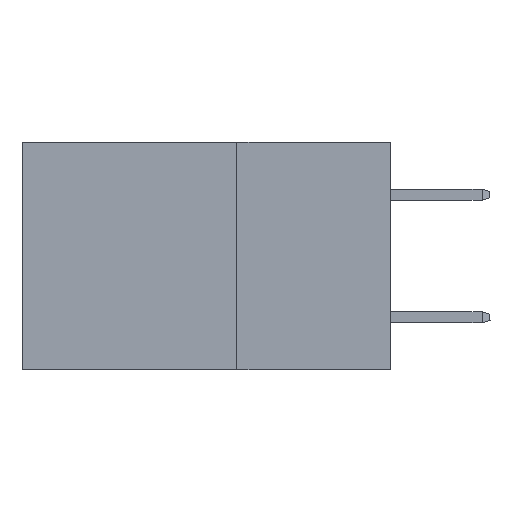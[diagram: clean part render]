
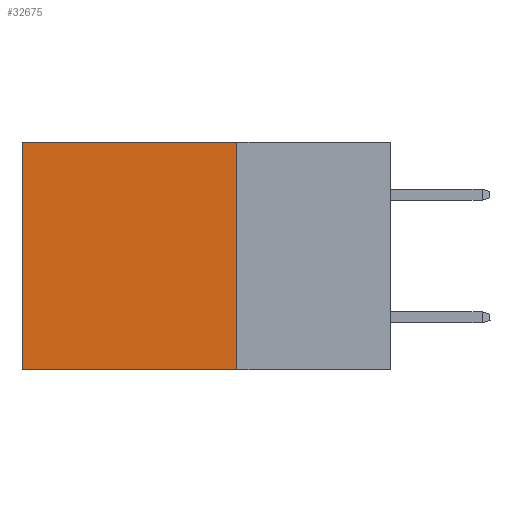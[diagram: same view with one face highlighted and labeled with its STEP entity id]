
A CAD part, left-side view. The second image highlights one B-rep face of the part: STEP entity #32675.
In plain terms, the highlighted planar face has unit normal (-1, 0, 0).
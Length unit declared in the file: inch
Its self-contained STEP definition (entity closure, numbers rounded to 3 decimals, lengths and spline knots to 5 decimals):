
#725 = DIRECTION ( 'NONE',  ( 0., 1., 0. ) ) ;
#2247 = CARTESIAN_POINT ( 'NONE',  ( 0.2875, 0.6, 0. ) ) ;
#2565 = CARTESIAN_POINT ( 'NONE',  ( 0.2875, 0.25, 0. ) ) ;
#4927 = VECTOR ( 'NONE', #38264, 39.37008 ) ;
#6407 = VECTOR ( 'NONE', #20916, 39.37008 ) ;
#6863 = CARTESIAN_POINT ( 'NONE',  ( 0.2875, 0.25, -0.37 ) ) ;
#7648 = ORIENTED_EDGE ( 'NONE', *, *, #24902, .T. ) ;
#8719 = VERTEX_POINT ( 'NONE', #2565 ) ;
#8982 = DIRECTION ( 'NONE',  ( 1., 0., 0. ) ) ;
#11031 = VERTEX_POINT ( 'NONE', #38211 ) ;
#12619 = CARTESIAN_POINT ( 'NONE',  ( 0.2875, 0.25, 0. ) ) ;
#19804 = ORIENTED_EDGE ( 'NONE', *, *, #27556, .T. ) ;
#20031 = CARTESIAN_POINT ( 'NONE',  ( 0.2875, 0.6, 0. ) ) ;
#20916 = DIRECTION ( 'NONE',  ( 0., 0., -1. ) ) ;
#21519 = VERTEX_POINT ( 'NONE', #20031 ) ;
#21698 = LINE ( 'NONE', #2247, #6407 ) ;
#22732 = LINE ( 'NONE', #6863, #33719 ) ;
#23766 = CARTESIAN_POINT ( 'NONE',  ( 0.2875, 0.25, -0.37 ) ) ;
#24271 = VECTOR ( 'NONE', #33984, 39.37008 ) ;
#24902 = EDGE_CURVE ( 'NONE', #21519, #11031, #21698, .T. ) ;
#27556 = EDGE_CURVE ( 'NONE', #8719, #21519, #37410, .T. ) ;
#27792 = ORIENTED_EDGE ( 'NONE', *, *, #37929, .F. ) ;
#29368 = ORIENTED_EDGE ( 'NONE', *, *, #31097, .F. ) ;
#31097 = EDGE_CURVE ( 'NONE', #8719, #38892, #32368, .T. ) ;
#31291 = EDGE_LOOP ( 'NONE', ( #7648, #27792, #29368, #19804 ) ) ;
#32368 = LINE ( 'NONE', #12619, #24271 ) ;
#32396 = CARTESIAN_POINT ( 'NONE',  ( 0.2875, 0.25, 0. ) ) ;
#32675 = ADVANCED_FACE ( 'NONE', ( #39393 ), #36250, .F. ) ;
#33719 = VECTOR ( 'NONE', #725, 39.37008 ) ;
#33984 = DIRECTION ( 'NONE',  ( 0., 0., -1. ) ) ;
#35988 = CARTESIAN_POINT ( 'NONE',  ( 0.2875, 0.25, 0. ) ) ;
#36250 = PLANE ( 'NONE',  #36838 ) ;
#36838 = AXIS2_PLACEMENT_3D ( 'NONE', #35988, #8982, #39296 ) ;
#37410 = LINE ( 'NONE', #32396, #4927 ) ;
#37929 = EDGE_CURVE ( 'NONE', #38892, #11031, #22732, .T. ) ;
#38211 = CARTESIAN_POINT ( 'NONE',  ( 0.2875, 0.6, -0.37 ) ) ;
#38264 = DIRECTION ( 'NONE',  ( 0., 1., 0. ) ) ;
#38892 = VERTEX_POINT ( 'NONE', #23766 ) ;
#39296 = DIRECTION ( 'NONE',  ( 0., 0., -1. ) ) ;
#39393 = FACE_OUTER_BOUND ( 'NONE', #31291, .T. ) ;
